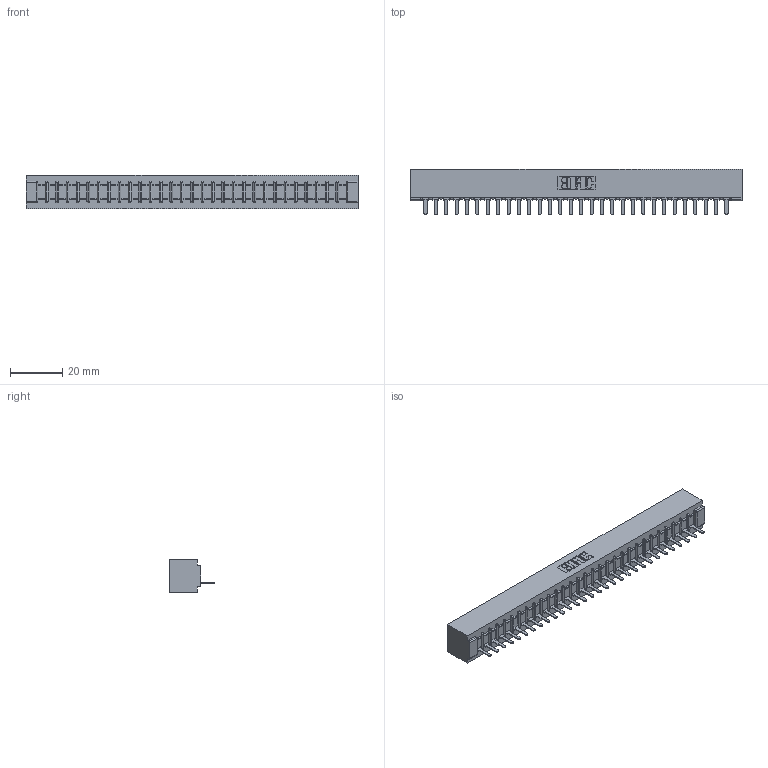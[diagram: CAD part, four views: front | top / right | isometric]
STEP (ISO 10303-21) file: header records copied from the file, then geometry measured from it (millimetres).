
FILE_DESCRIPTION (( 'STEP AP203' ), '1' );
FILE_NAME ('307-030-521-101.STEP', '2018-08-04T18:56:43', ( '' ), ( '' ), 'SwSTEP 2.0', 'SolidWorks 2016', '' );
FILE_SCHEMA (( 'CONFIG_CONTROL_DESIGN' ));
Length unit declared in the file: inch
Products named in the file (3): 307 Part_No Mounting Lugs; 307-290-002_521; 307-030-521-101
Assembly tree (31 placements, depth 2):
  307-030-521-101
    307 Part_No Mounting Lugs
    307-290-002_521  x30
Bounding box: 126.75 x 17.42 x 12.7 mm (x, y, z)
Volume: 14033.5 mm3; surface area: 17737.1 mm2
Topology: 31 solids, 31 shells, 2361 faces, 7259 edges, 4754 vertices
Faces by surface type: plane 1416, cylinder 883, sphere 62
Entity records: 27638 total; most frequent: CARTESIAN_POINT 4660, ORIENTED_EDGE 4650, DIRECTION 4531, EDGE_CURVE 2325, VECTOR 1777, LINE 1777, VERTEX_POINT 1506, AXIS2_PLACEMENT_3D 1377
